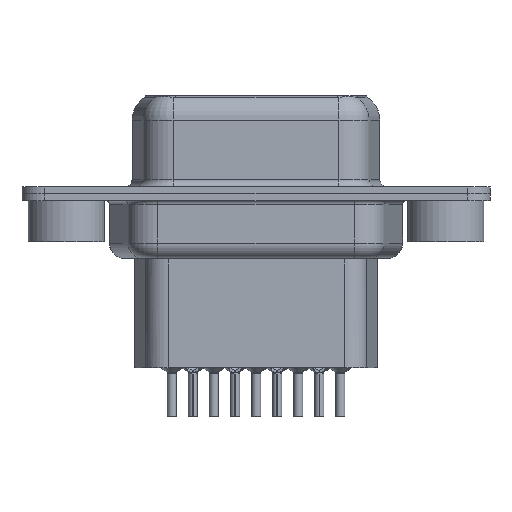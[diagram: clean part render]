
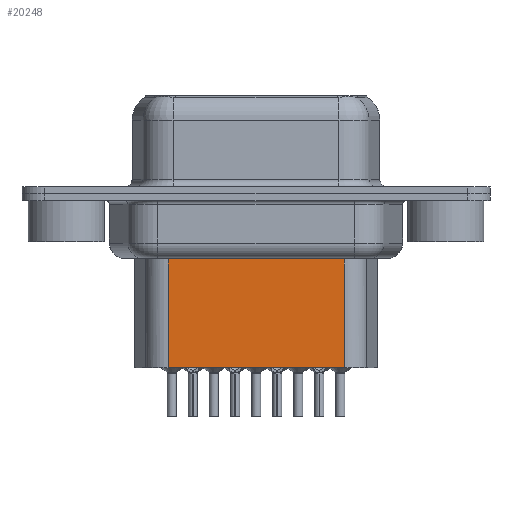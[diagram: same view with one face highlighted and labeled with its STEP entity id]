
A CAD part, front view. The second image highlights one B-rep face of the part: STEP entity #20248.
In plain terms, the highlighted planar face has unit normal (0, -1, 0).
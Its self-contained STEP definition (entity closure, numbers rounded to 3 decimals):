
#23 = CARTESIAN_POINT ( 'NONE',  ( 18.294, -3.5, -4.097 ) ) ;
#114 = PLANE ( 'NONE',  #18191 ) ;
#1840 = DIRECTION ( 'NONE',  ( 1., 0., 0. ) ) ;
#2239 = LINE ( 'NONE', #10908, #15069 ) ;
#4540 = ORIENTED_EDGE ( 'NONE', *, *, #10653, .F. ) ;
#5638 = EDGE_CURVE ( 'NONE', #15087, #14261, #2239, .T. ) ;
#7248 = DIRECTION ( 'NONE',  ( 0., 0., -1. ) ) ;
#7632 = CARTESIAN_POINT ( 'NONE',  ( 6.459, -3.5, -4.097 ) ) ;
#7804 = DIRECTION ( 'NONE',  ( 0., 0., -1. ) ) ;
#8650 = CARTESIAN_POINT ( 'NONE',  ( 6.706, -3.5, -4.097 ) ) ;
#10026 = CARTESIAN_POINT ( 'NONE',  ( 6.706, -3.5, -3.1 ) ) ;
#10653 = EDGE_CURVE ( 'NONE', #12108, #15087, #21388, .T. ) ;
#10908 = CARTESIAN_POINT ( 'NONE',  ( 6.706, -3.5, -11.45 ) ) ;
#10979 = DIRECTION ( 'NONE',  ( -1., 0., 0. ) ) ;
#11813 = ORIENTED_EDGE ( 'NONE', *, *, #14486, .T. ) ;
#11933 = DIRECTION ( 'NONE',  ( 0., -1., 0. ) ) ;
#11957 = CARTESIAN_POINT ( 'NONE',  ( 6.706, -3.5, -11.45 ) ) ;
#12108 = VERTEX_POINT ( 'NONE', #23 ) ;
#12235 = CARTESIAN_POINT ( 'NONE',  ( 18.294, -3.5, -3.1 ) ) ;
#12930 = ORIENTED_EDGE ( 'NONE', *, *, #5638, .F. ) ;
#13227 = CARTESIAN_POINT ( 'NONE',  ( 18.294, -3.5, -11.45 ) ) ;
#13980 = EDGE_CURVE ( 'NONE', #14655, #14261, #15635, .T. ) ;
#14261 = VERTEX_POINT ( 'NONE', #11957 ) ;
#14486 = EDGE_CURVE ( 'NONE', #12108, #14655, #14799, .T. ) ;
#14655 = VERTEX_POINT ( 'NONE', #8650 ) ;
#14799 = LINE ( 'NONE', #7632, #18646 ) ;
#15069 = VECTOR ( 'NONE', #10979, 1000. ) ;
#15087 = VERTEX_POINT ( 'NONE', #13227 ) ;
#15211 = EDGE_LOOP ( 'NONE', ( #4540, #11813, #18858, #12930 ) ) ;
#15635 = LINE ( 'NONE', #19381, #19487 ) ;
#15968 = VECTOR ( 'NONE', #7248, 1000. ) ;
#17564 = DIRECTION ( 'NONE',  ( -1., 0., 0. ) ) ;
#18191 = AXIS2_PLACEMENT_3D ( 'NONE', #10026, #11933, #1840 ) ;
#18646 = VECTOR ( 'NONE', #17564, 1000. ) ;
#18858 = ORIENTED_EDGE ( 'NONE', *, *, #13980, .T. ) ;
#19381 = CARTESIAN_POINT ( 'NONE',  ( 6.706, -3.5, -3.1 ) ) ;
#19487 = VECTOR ( 'NONE', #7804, 1000. ) ;
#20248 = ADVANCED_FACE ( 'NONE', ( #21306 ), #114, .T. ) ;
#21306 = FACE_OUTER_BOUND ( 'NONE', #15211, .T. ) ;
#21388 = LINE ( 'NONE', #12235, #15968 ) ;
